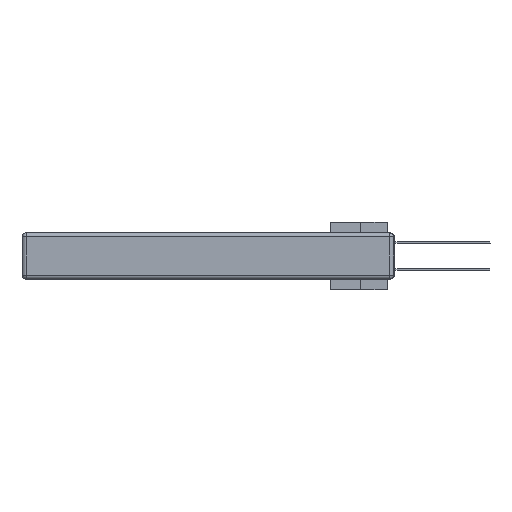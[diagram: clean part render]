
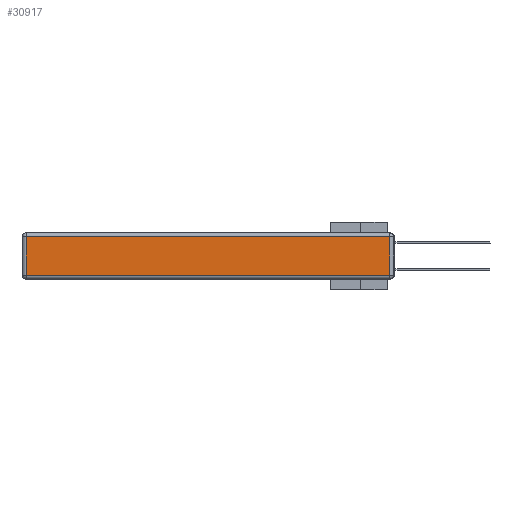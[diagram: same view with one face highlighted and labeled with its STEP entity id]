
A CAD part, left-side view. The second image highlights one B-rep face of the part: STEP entity #30917.
In plain terms, the highlighted planar face has unit normal (-1, 0, 0).
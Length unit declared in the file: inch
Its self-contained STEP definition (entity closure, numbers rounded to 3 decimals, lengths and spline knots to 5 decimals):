
#751 = LINE ( 'NONE', #16791, #29100 ) ;
#922 = CARTESIAN_POINT ( 'NONE',  ( 0., 0., -0.313 ) ) ;
#1898 = EDGE_CURVE ( 'NONE', #8759, #33835, #751, .T. ) ;
#4756 = ORIENTED_EDGE ( 'NONE', *, *, #33065, .T. ) ;
#5395 = EDGE_LOOP ( 'NONE', ( #4756, #26844, #14108, #18482 ) ) ;
#5988 = DIRECTION ( 'NONE',  ( 0., 0., 1. ) ) ;
#7537 = VECTOR ( 'NONE', #16938, 39.37008 ) ;
#8759 = VERTEX_POINT ( 'NONE', #26873 ) ;
#9793 = VERTEX_POINT ( 'NONE', #22489 ) ;
#9822 = CARTESIAN_POINT ( 'NONE',  ( 0., 0., -0.343 ) ) ;
#12259 = LINE ( 'NONE', #22567, #7537 ) ;
#12563 = DIRECTION ( 'NONE',  ( -1., 0., 0. ) ) ;
#13954 = LINE ( 'NONE', #922, #35378 ) ;
#14108 = ORIENTED_EDGE ( 'NONE', *, *, #25441, .T. ) ;
#14733 = DIRECTION ( 'NONE',  ( 0., -1., 0. ) ) ;
#15369 = DIRECTION ( 'NONE',  ( 0., 0., 1. ) ) ;
#15709 = CARTESIAN_POINT ( 'NONE',  ( 0., 2.72, -0.343 ) ) ;
#15836 = DIRECTION ( 'NONE',  ( 0., 0., -1. ) ) ;
#16791 = CARTESIAN_POINT ( 'NONE',  ( 0., 0.03, -0.343 ) ) ;
#16938 = DIRECTION ( 'NONE',  ( 0., 1., 0. ) ) ;
#18482 = ORIENTED_EDGE ( 'NONE', *, *, #20796, .T. ) ;
#20796 = EDGE_CURVE ( 'NONE', #29694, #9793, #25072, .T. ) ;
#22489 = CARTESIAN_POINT ( 'NONE',  ( 0., 2.72, -0.313 ) ) ;
#22567 = CARTESIAN_POINT ( 'NONE',  ( 0., 2.75, -0.03 ) ) ;
#24933 = CARTESIAN_POINT ( 'NONE',  ( 0., 0.03, -0.03 ) ) ;
#25072 = LINE ( 'NONE', #15709, #30232 ) ;
#25441 = EDGE_CURVE ( 'NONE', #33835, #29694, #12259, .T. ) ;
#26193 = CARTESIAN_POINT ( 'NONE',  ( 0., 2.72, -0.03 ) ) ;
#26616 = PLANE ( 'NONE',  #31141 ) ;
#26844 = ORIENTED_EDGE ( 'NONE', *, *, #1898, .T. ) ;
#26873 = CARTESIAN_POINT ( 'NONE',  ( 0., 0.03, -0.313 ) ) ;
#29100 = VECTOR ( 'NONE', #5988, 39.37008 ) ;
#29694 = VERTEX_POINT ( 'NONE', #26193 ) ;
#30232 = VECTOR ( 'NONE', #15836, 39.37008 ) ;
#30917 = ADVANCED_FACE ( 'NONE', ( #34451 ), #26616, .T. ) ;
#31141 = AXIS2_PLACEMENT_3D ( 'NONE', #9822, #12563, #15369 ) ;
#33065 = EDGE_CURVE ( 'NONE', #9793, #8759, #13954, .T. ) ;
#33835 = VERTEX_POINT ( 'NONE', #24933 ) ;
#34451 = FACE_OUTER_BOUND ( 'NONE', #5395, .T. ) ;
#35378 = VECTOR ( 'NONE', #14733, 39.37008 ) ;
